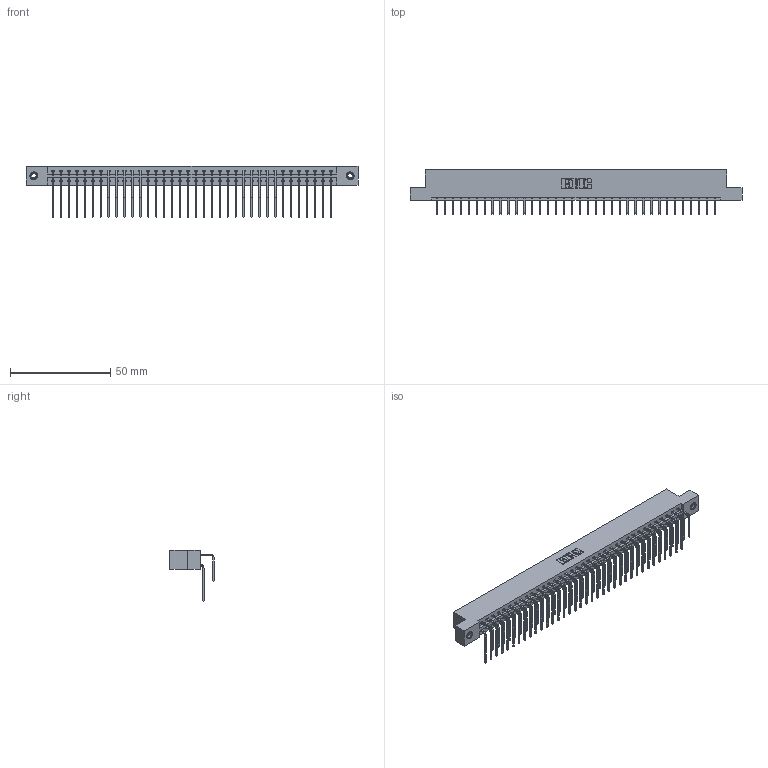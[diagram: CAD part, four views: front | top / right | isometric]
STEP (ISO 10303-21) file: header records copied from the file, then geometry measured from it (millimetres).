
FILE_DESCRIPTION (( 'STEP AP203' ), '1' );
FILE_NAME ('387-072-558-208.STEP', '2019-10-22T00:38:03', ( '' ), ( '' ), 'SwSTEP 2.0', 'SolidWorks 2016', '' );
FILE_SCHEMA (( 'CONFIG_CONTROL_DESIGN' ));
Length unit declared in the file: inch
Products named in the file (5): 345-292-001_558 Tail - 2; 387-072-558-208; 345-250-001_345-250-003-102; 337 Part_Flush Mounting Lugs - 0.156 Dia-TI; 345-292-001_558 559 Tail - 1
Assembly tree (75 placements, depth 2):
  387-072-558-208
    337 Part_Flush Mounting Lugs - 0.156 Dia-TI
    345-292-001_558 559 Tail - 1  x36
    345-292-001_558 Tail - 2  x36
    345-250-001_345-250-003-102  x2
Bounding box: 165.66 x 22.17 x 25.53 mm (x, y, z)
Volume: 17787.4 mm3; surface area: 22159.9 mm2
Topology: 75 solids, 75 shells, 4206 faces, 12471 edges, 8210 vertices
Faces by surface type: plane 2982, cylinder 1208, cone 12, torus 4
Entity records: 31658 total; most frequent: CARTESIAN_POINT 5364, ORIENTED_EDGE 5242, DIRECTION 4587, EDGE_CURVE 2621, LINE 2433, VECTOR 2433, VERTEX_POINT 1740, AXIS2_PLACEMENT_3D 1077
